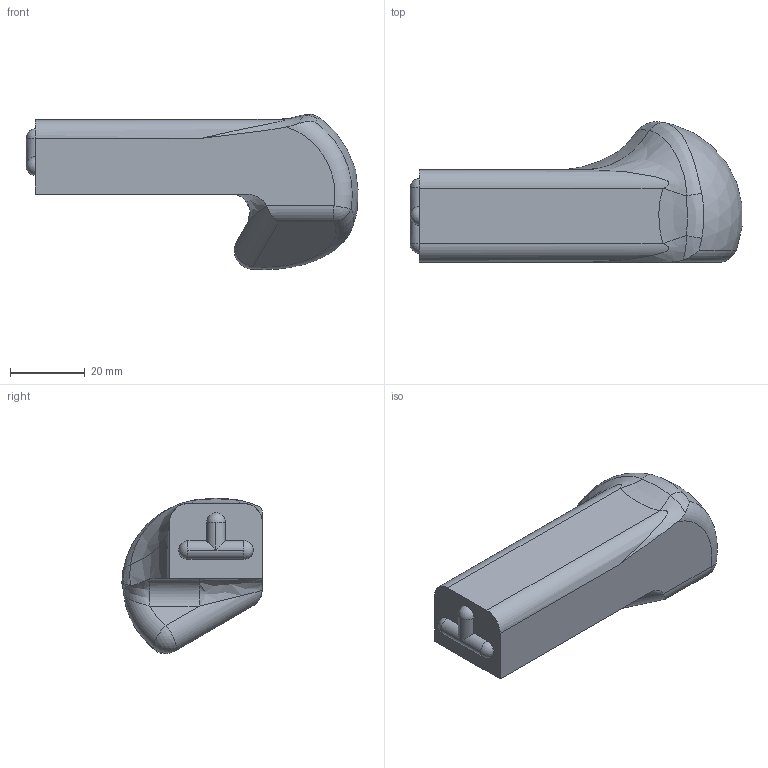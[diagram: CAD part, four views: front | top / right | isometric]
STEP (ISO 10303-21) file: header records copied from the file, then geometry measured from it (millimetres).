
FILE_DESCRIPTION (( 'STEP AP214' ), '1' );
FILE_NAME ('Bipod_Left_Part_1_V2.step', '2016-01-25T18:17:10', ( 'WarFairy' ), ( '' ), 'SwSTEP 2.0', 'SolidWorks 2015', '' );
FILE_SCHEMA (( 'AUTOMOTIVE_DESIGN' ));
Length unit declared in the file: millimetre
Products named in the file (1): Bipod_Left_Part_1_V2
Bounding box: 88.96 x 37.62 x 41.6 mm (x, y, z)
Volume: 55809.1 mm3; surface area: 9785.9 mm2
Topology: 1 solids, 1 shells, 37 faces, 92 edges, 54 vertices
Faces by surface type: bspline 11, cylinder 10, plane 7, sphere 6, torus 3
Entity records: 1851 total; most frequent: CARTESIAN_POINT 1066, ORIENTED_EDGE 170, DIRECTION 140, EDGE_CURVE 85, AXIS2_PLACEMENT_3D 58, VERTEX_POINT 51, EDGE_LOOP 38, ADVANCED_FACE 37
